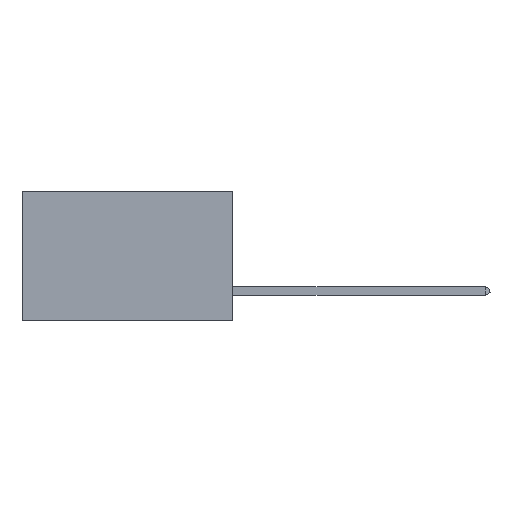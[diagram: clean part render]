
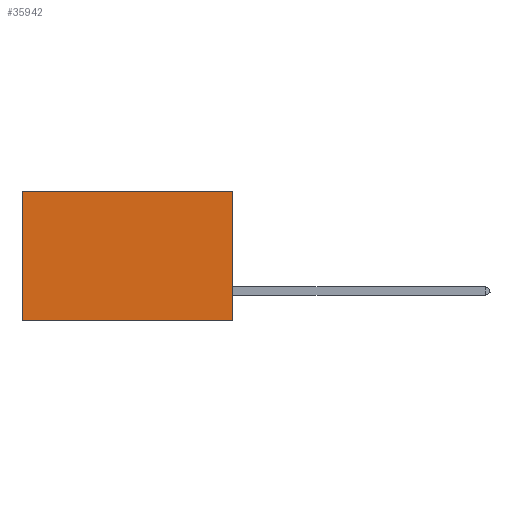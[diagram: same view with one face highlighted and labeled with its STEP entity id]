
A CAD part, left-side view. The second image highlights one B-rep face of the part: STEP entity #35942.
In plain terms, the highlighted planar face has unit normal (-1, 0, 0).
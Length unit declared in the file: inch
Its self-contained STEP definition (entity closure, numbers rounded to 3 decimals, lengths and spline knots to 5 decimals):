
#2996 = CARTESIAN_POINT ( 'NONE',  ( 0.2875, 0.6, -0.37 ) ) ;
#3001 = CARTESIAN_POINT ( 'NONE',  ( 0.2875, 0., 0. ) ) ;
#3295 = CARTESIAN_POINT ( 'NONE',  ( 0.2875, 0.6, 0. ) ) ;
#4769 = CARTESIAN_POINT ( 'NONE',  ( 0.2875, 0., -0.37 ) ) ;
#4976 = LINE ( 'NONE', #16977, #16921 ) ;
#5262 = DIRECTION ( 'NONE',  ( 0., 1., 0. ) ) ;
#6097 = EDGE_LOOP ( 'NONE', ( #20882, #8547, #14454, #16631 ) ) ;
#6198 = EDGE_CURVE ( 'NONE', #10084, #12499, #4976, .T. ) ;
#7145 = DIRECTION ( 'NONE',  ( 0., 0., -1. ) ) ;
#8547 = ORIENTED_EDGE ( 'NONE', *, *, #28053, .F. ) ;
#10084 = VERTEX_POINT ( 'NONE', #16253 ) ;
#12499 = VERTEX_POINT ( 'NONE', #3295 ) ;
#12843 = VERTEX_POINT ( 'NONE', #36775 ) ;
#13419 = AXIS2_PLACEMENT_3D ( 'NONE', #3001, #27464, #31931 ) ;
#13421 = LINE ( 'NONE', #15887, #29107 ) ;
#14454 = ORIENTED_EDGE ( 'NONE', *, *, #17939, .F. ) ;
#14800 = FACE_OUTER_BOUND ( 'NONE', #6097, .T. ) ;
#15887 = CARTESIAN_POINT ( 'NONE',  ( 0.2875, 0.6, 0. ) ) ;
#16253 = CARTESIAN_POINT ( 'NONE',  ( 0.2875, 0., 0. ) ) ;
#16631 = ORIENTED_EDGE ( 'NONE', *, *, #6198, .T. ) ;
#16921 = VECTOR ( 'NONE', #5262, 39.37008 ) ;
#16977 = CARTESIAN_POINT ( 'NONE',  ( 0.2875, 0., 0. ) ) ;
#16986 = DIRECTION ( 'NONE',  ( 0., 1., 0. ) ) ;
#17939 = EDGE_CURVE ( 'NONE', #10084, #12843, #37021, .T. ) ;
#18868 = EDGE_CURVE ( 'NONE', #12499, #24278, #13421, .T. ) ;
#18889 = CARTESIAN_POINT ( 'NONE',  ( 0.2875, 0., 0. ) ) ;
#20442 = VECTOR ( 'NONE', #16986, 39.37008 ) ;
#20882 = ORIENTED_EDGE ( 'NONE', *, *, #18868, .T. ) ;
#21844 = DIRECTION ( 'NONE',  ( 0., 0., -1. ) ) ;
#24278 = VERTEX_POINT ( 'NONE', #2996 ) ;
#24443 = PLANE ( 'NONE',  #13419 ) ;
#25047 = VECTOR ( 'NONE', #7145, 39.37008 ) ;
#27464 = DIRECTION ( 'NONE',  ( 1., 0., 0. ) ) ;
#28053 = EDGE_CURVE ( 'NONE', #12843, #24278, #28314, .T. ) ;
#28314 = LINE ( 'NONE', #4769, #20442 ) ;
#29107 = VECTOR ( 'NONE', #21844, 39.37008 ) ;
#31931 = DIRECTION ( 'NONE',  ( 0., 0., -1. ) ) ;
#35942 = ADVANCED_FACE ( 'NONE', ( #14800 ), #24443, .F. ) ;
#36775 = CARTESIAN_POINT ( 'NONE',  ( 0.2875, 0., -0.37 ) ) ;
#37021 = LINE ( 'NONE', #18889, #25047 ) ;
